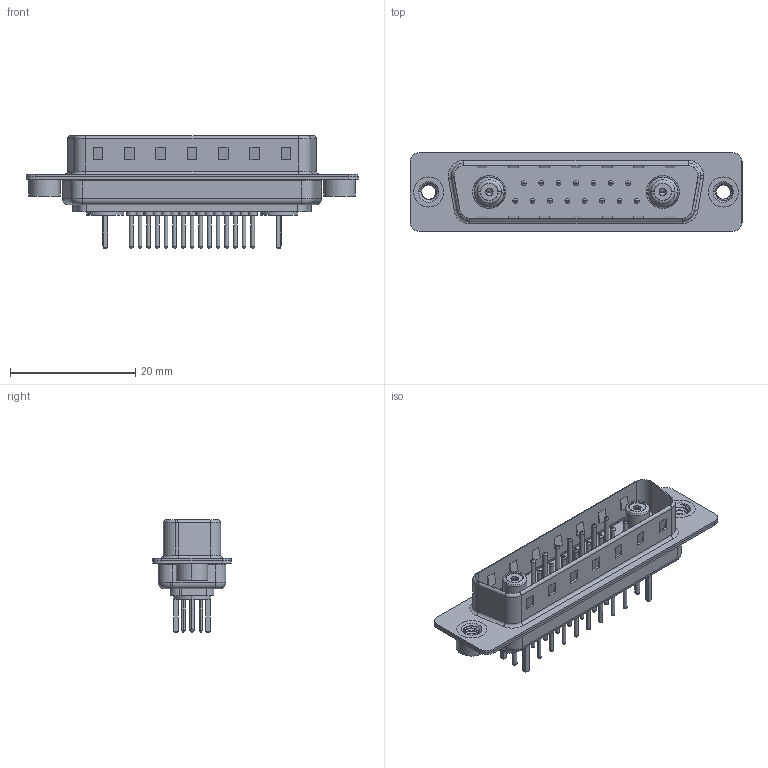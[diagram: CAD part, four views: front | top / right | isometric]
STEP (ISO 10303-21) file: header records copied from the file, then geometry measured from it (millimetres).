
FILE_DESCRIPTION (( 'STEP AP203' ), '1' );
FILE_NAME ('627-17W2624-5TA.STEP', '2019-05-27T23:09:41', ( '' ), ( '' ), 'SwSTEP 2.0', 'SolidWorks 2016', '' );
FILE_SCHEMA (( 'CONFIG_CONTROL_DESIGN' ));
Length unit declared in the file: millimetre
Products named in the file (14): 627Combo Shell Rear_25 Contacts; Locking Collar; Insulator Socket; Socket_Str; 627Combo Housing_17W2; 627Combo Contact Row 1_24; 627Combo Shell Front_25 Contacts; 627Combo Threaded Rivet_2; Insulator Socket 2; Co-Ax Jack_Straight PC Tail; 627Combo Threaded Rivet_A; 627Combo Contact Row 2_24; Co-Ax Jack Assy_S; 627-17W2624-5TA
Assembly tree (27 placements, depth 3):
  627-17W2624-5TA
    627Combo Housing_17W2
    627Combo Shell Rear_25 Contacts
    627Combo Shell Front_25 Contacts
    627Combo Threaded Rivet_A
    Co-Ax Jack Assy_S  x2
      Co-Ax Jack_Straight PC Tail
      Insulator Socket
      Insulator Socket 2
      Locking Collar
      Socket_Str
    627Combo Threaded Rivet_2
    627Combo Contact Row 1_24  x7
    627Combo Contact Row 2_24  x8
Bounding box: 53 x 12.6 x 17.9 mm (x, y, z)
Volume: 2762.7 mm3; surface area: 7596.4 mm2
Topology: 30 solids, 30 shells, 1152 faces, 2562 edges, 1572 vertices
Faces by surface type: cylinder 442, plane 370, torus 298, cone 28, bspline 10, sphere 4
Entity records: 24697 total; most frequent: CARTESIAN_POINT 6729, DIRECTION 3603, ORIENTED_EDGE 3182, EDGE_CURVE 1591, AXIS2_PLACEMENT_3D 1411, VERTEX_POINT 1008, EDGE_LOOP 815, VECTOR 781
